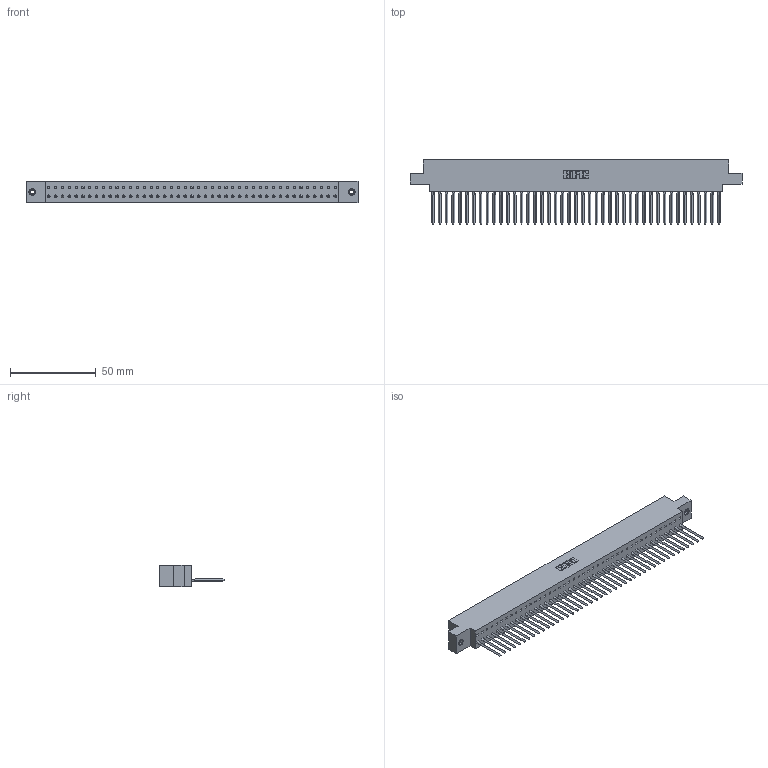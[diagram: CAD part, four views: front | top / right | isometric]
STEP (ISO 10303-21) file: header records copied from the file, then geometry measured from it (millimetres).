
FILE_DESCRIPTION (( 'STEP AP203' ), '1' );
FILE_NAME ('317-043-541-608.STEP', '2020-02-28T01:53:48', ( '' ), ( '' ), 'SwSTEP 2.0', 'SolidWorks 2016', '' );
FILE_SCHEMA (( 'CONFIG_CONTROL_DESIGN' ));
Length unit declared in the file: inch
Products named in the file (4): 317 Part_.156 Dia - TI; 317-043-541-608; 345-250-001_345-250-003-102; 317-290-002_541
Assembly tree (46 placements, depth 2):
  317-043-541-608
    317 Part_.156 Dia - TI
    317-290-002_541  x43
    345-250-001_345-250-003-102  x2
Bounding box: 193.09 x 37.34 x 12.7 mm (x, y, z)
Volume: 31337.1 mm3; surface area: 44336.2 mm2
Topology: 46 solids, 46 shells, 6698 faces, 19073 edges, 12392 vertices
Faces by surface type: plane 5422, cylinder 1088, bspline 172, cone 12, torus 4
Entity records: 63375 total; most frequent: CARTESIAN_POINT 11877, ORIENTED_EDGE 11166, DIRECTION 9215, EDGE_CURVE 5583, LINE 5199, VECTOR 5199, VERTEX_POINT 3710, AXIS2_PLACEMENT_3D 2008
